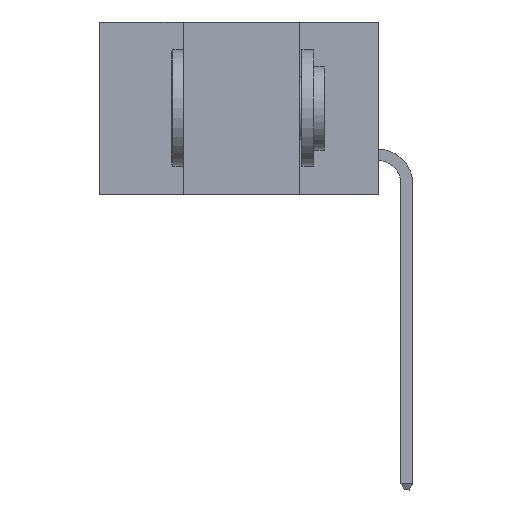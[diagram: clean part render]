
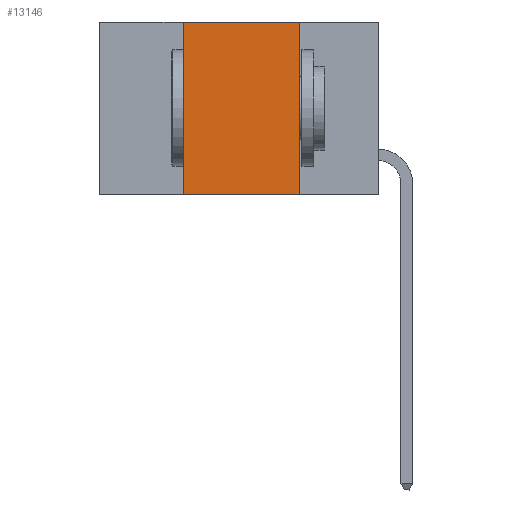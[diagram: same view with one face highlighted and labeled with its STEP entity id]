
A CAD part, left-side view. The second image highlights one B-rep face of the part: STEP entity #13146.
In plain terms, the highlighted planar face has unit normal (-1, 0, 0).
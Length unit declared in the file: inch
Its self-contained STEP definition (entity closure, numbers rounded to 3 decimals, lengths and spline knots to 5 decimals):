
#651 = VERTEX_POINT ( 'NONE', #4426 ) ;
#1116 = VECTOR ( 'NONE', #1260, 39.37008 ) ;
#1235 = ORIENTED_EDGE ( 'NONE', *, *, #13420, .T. ) ;
#1260 = DIRECTION ( 'NONE',  ( 0., -1., 0. ) ) ;
#1289 = EDGE_LOOP ( 'NONE', ( #13040, #15934, #2633, #1235 ) ) ;
#1820 = EDGE_CURVE ( 'NONE', #10669, #7882, #8385, .T. ) ;
#2633 = ORIENTED_EDGE ( 'NONE', *, *, #7966, .F. ) ;
#3340 = FACE_OUTER_BOUND ( 'NONE', #1289, .T. ) ;
#4426 = CARTESIAN_POINT ( 'NONE',  ( 0., 0.42, 0. ) ) ;
#4518 = LINE ( 'NONE', #8723, #1116 ) ;
#5136 = VECTOR ( 'NONE', #5905, 39.37008 ) ;
#5609 = CARTESIAN_POINT ( 'NONE',  ( 0., 0.17, 0. ) ) ;
#5641 = LINE ( 'NONE', #11394, #8896 ) ;
#5825 = DIRECTION ( 'NONE',  ( 0., 0., -1. ) ) ;
#5905 = DIRECTION ( 'NONE',  ( 0., 0., -1. ) ) ;
#5979 = CARTESIAN_POINT ( 'NONE',  ( 0., 0.42, -0.37 ) ) ;
#6053 = CARTESIAN_POINT ( 'NONE',  ( 0., 0.42, 0. ) ) ;
#6191 = DIRECTION ( 'NONE',  ( 0., 0., 1. ) ) ;
#7142 = CARTESIAN_POINT ( 'NONE',  ( 0., 0.17, -0.37 ) ) ;
#7882 = VERTEX_POINT ( 'NONE', #7142 ) ;
#7966 = EDGE_CURVE ( 'NONE', #11156, #651, #9357, .T. ) ;
#8385 = LINE ( 'NONE', #10080, #5136 ) ;
#8723 = CARTESIAN_POINT ( 'NONE',  ( 0., 0.6, 0. ) ) ;
#8896 = VECTOR ( 'NONE', #10148, 39.37008 ) ;
#9357 = LINE ( 'NONE', #6053, #15949 ) ;
#10080 = CARTESIAN_POINT ( 'NONE',  ( 0., 0.17, 0. ) ) ;
#10148 = DIRECTION ( 'NONE',  ( 0., -1., 0. ) ) ;
#10669 = VERTEX_POINT ( 'NONE', #5609 ) ;
#10676 = PLANE ( 'NONE',  #13822 ) ;
#11156 = VERTEX_POINT ( 'NONE', #5979 ) ;
#11394 = CARTESIAN_POINT ( 'NONE',  ( 0., 0.6, -0.37 ) ) ;
#11928 = CARTESIAN_POINT ( 'NONE',  ( 0., 0.6, 0. ) ) ;
#13040 = ORIENTED_EDGE ( 'NONE', *, *, #1820, .F. ) ;
#13146 = ADVANCED_FACE ( 'NONE', ( #3340 ), #10676, .F. ) ;
#13189 = DIRECTION ( 'NONE',  ( 1., 0., 0. ) ) ;
#13420 = EDGE_CURVE ( 'NONE', #11156, #7882, #5641, .T. ) ;
#13822 = AXIS2_PLACEMENT_3D ( 'NONE', #11928, #13189, #5825 ) ;
#15328 = EDGE_CURVE ( 'NONE', #651, #10669, #4518, .T. ) ;
#15934 = ORIENTED_EDGE ( 'NONE', *, *, #15328, .F. ) ;
#15949 = VECTOR ( 'NONE', #6191, 39.37008 ) ;
